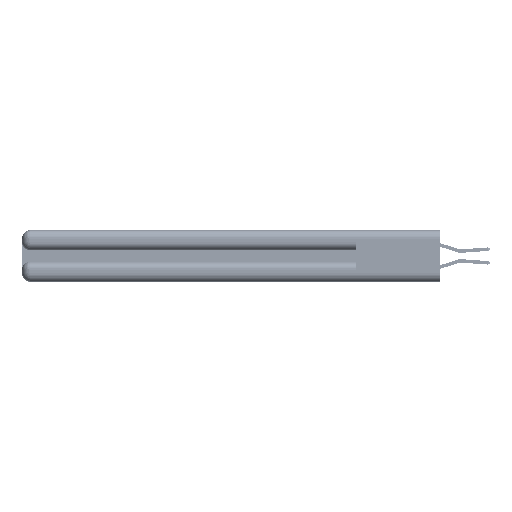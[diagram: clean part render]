
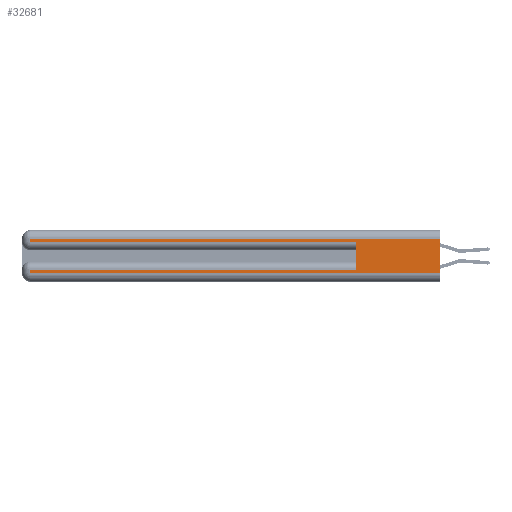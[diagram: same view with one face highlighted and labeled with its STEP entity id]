
A CAD part, left-side view. The second image highlights one B-rep face of the part: STEP entity #32681.
In plain terms, the highlighted planar face has unit normal (-1, 0, 0).
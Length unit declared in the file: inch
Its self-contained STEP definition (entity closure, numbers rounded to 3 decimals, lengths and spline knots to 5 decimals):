
#634 = VECTOR ( 'NONE', #20663, 39.37008 ) ;
#1215 = ORIENTED_EDGE ( 'NONE', *, *, #43370, .T. ) ;
#1326 = LINE ( 'NONE', #36143, #11217 ) ;
#4264 = VECTOR ( 'NONE', #19446, 39.37008 ) ;
#4294 = ORIENTED_EDGE ( 'NONE', *, *, #17180, .T. ) ;
#5537 = FACE_OUTER_BOUND ( 'NONE', #32878, .T. ) ;
#5872 = EDGE_CURVE ( 'NONE', #7615, #18697, #41467, .T. ) ;
#7209 = LINE ( 'NONE', #17438, #46704 ) ;
#7463 = EDGE_CURVE ( 'NONE', #13482, #46903, #34678, .T. ) ;
#7615 = VERTEX_POINT ( 'NONE', #15933 ) ;
#8559 = LINE ( 'NONE', #41062, #634 ) ;
#8847 = CARTESIAN_POINT ( 'NONE',  ( 0., 0., 0.06 ) ) ;
#8947 = DIRECTION ( 'NONE',  ( 0., -1., 0. ) ) ;
#9168 = LINE ( 'NONE', #8847, #21705 ) ;
#9787 = CARTESIAN_POINT ( 'NONE',  ( 0., 0.6, 0.085 ) ) ;
#9913 = DIRECTION ( 'NONE',  ( 0., 0., 1. ) ) ;
#10181 = ORIENTED_EDGE ( 'NONE', *, *, #7463, .F. ) ;
#10541 = CARTESIAN_POINT ( 'NONE',  ( 0., 0., 0.37 ) ) ;
#11122 = CARTESIAN_POINT ( 'NONE',  ( 0., 2.94, 0.31 ) ) ;
#11217 = VECTOR ( 'NONE', #45143, 39.37008 ) ;
#11936 = ORIENTED_EDGE ( 'NONE', *, *, #43352, .T. ) ;
#12779 = CARTESIAN_POINT ( 'NONE',  ( 0., 0., 0.06 ) ) ;
#13482 = VERTEX_POINT ( 'NONE', #9787 ) ;
#15289 = AXIS2_PLACEMENT_3D ( 'NONE', #43210, #25912, #30141 ) ;
#15468 = LINE ( 'NONE', #31412, #4264 ) ;
#15933 = CARTESIAN_POINT ( 'NONE',  ( 0., 0., 0.31 ) ) ;
#17180 = EDGE_CURVE ( 'NONE', #49903, #42789, #9168, .T. ) ;
#17191 = CARTESIAN_POINT ( 'NONE',  ( 0., 2.94, 0.085 ) ) ;
#17438 = CARTESIAN_POINT ( 'NONE',  ( 0., 0., 0.285 ) ) ;
#18697 = VERTEX_POINT ( 'NONE', #11122 ) ;
#19363 = VERTEX_POINT ( 'NONE', #20065 ) ;
#19446 = DIRECTION ( 'NONE',  ( 0., 1., 0. ) ) ;
#20065 = CARTESIAN_POINT ( 'NONE',  ( 0., 2.94, 0.285 ) ) ;
#20663 = DIRECTION ( 'NONE',  ( 0., 0., -1. ) ) ;
#21705 = VECTOR ( 'NONE', #42710, 39.37008 ) ;
#22658 = VERTEX_POINT ( 'NONE', #17191 ) ;
#23395 = EDGE_CURVE ( 'NONE', #19363, #46903, #7209, .T. ) ;
#25313 = ORIENTED_EDGE ( 'NONE', *, *, #23395, .T. ) ;
#25912 = DIRECTION ( 'NONE',  ( 1., 0., 0. ) ) ;
#26650 = CARTESIAN_POINT ( 'NONE',  ( 0., 0.6, 0.145 ) ) ;
#30141 = DIRECTION ( 'NONE',  ( 0., 0., -1. ) ) ;
#31412 = CARTESIAN_POINT ( 'NONE',  ( 0., 0., 0.085 ) ) ;
#32681 = ADVANCED_FACE ( 'NONE', ( #5537 ), #42846, .F. ) ;
#32878 = EDGE_LOOP ( 'NONE', ( #52328, #40526, #1215, #25313, #10181, #53879, #11936, #4294 ) ) ;
#34678 = LINE ( 'NONE', #26650, #52453 ) ;
#36143 = CARTESIAN_POINT ( 'NONE',  ( 0., 2.94, 0.37 ) ) ;
#39384 = CARTESIAN_POINT ( 'NONE',  ( 0., 0.6, 0.285 ) ) ;
#40410 = DIRECTION ( 'NONE',  ( 0., 1., 0. ) ) ;
#40526 = ORIENTED_EDGE ( 'NONE', *, *, #5872, .T. ) ;
#41062 = CARTESIAN_POINT ( 'NONE',  ( 0., 2.94, 0.37 ) ) ;
#41467 = LINE ( 'NONE', #48706, #42795 ) ;
#42710 = DIRECTION ( 'NONE',  ( 0., -1., 0. ) ) ;
#42789 = VERTEX_POINT ( 'NONE', #12779 ) ;
#42795 = VECTOR ( 'NONE', #40410, 39.37008 ) ;
#42846 = PLANE ( 'NONE',  #15289 ) ;
#43210 = CARTESIAN_POINT ( 'NONE',  ( 0., 0., 0.37 ) ) ;
#43352 = EDGE_CURVE ( 'NONE', #22658, #49903, #1326, .T. ) ;
#43370 = EDGE_CURVE ( 'NONE', #18697, #19363, #8559, .T. ) ;
#45143 = DIRECTION ( 'NONE',  ( 0., 0., -1. ) ) ;
#45255 = LINE ( 'NONE', #10541, #47892 ) ;
#46401 = EDGE_CURVE ( 'NONE', #7615, #42789, #45255, .T. ) ;
#46704 = VECTOR ( 'NONE', #8947, 39.37008 ) ;
#46903 = VERTEX_POINT ( 'NONE', #39384 ) ;
#47814 = EDGE_CURVE ( 'NONE', #13482, #22658, #15468, .T. ) ;
#47892 = VECTOR ( 'NONE', #48441, 39.37008 ) ;
#48441 = DIRECTION ( 'NONE',  ( 0., 0., -1. ) ) ;
#48706 = CARTESIAN_POINT ( 'NONE',  ( 0., 0., 0.31 ) ) ;
#49903 = VERTEX_POINT ( 'NONE', #51115 ) ;
#51115 = CARTESIAN_POINT ( 'NONE',  ( 0., 2.94, 0.06 ) ) ;
#52328 = ORIENTED_EDGE ( 'NONE', *, *, #46401, .F. ) ;
#52453 = VECTOR ( 'NONE', #9913, 39.37008 ) ;
#53879 = ORIENTED_EDGE ( 'NONE', *, *, #47814, .T. ) ;
